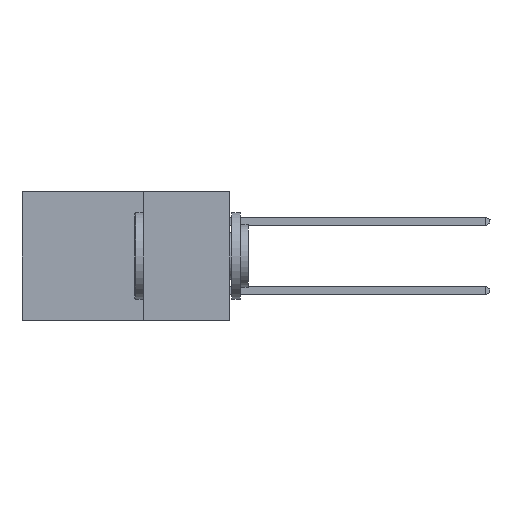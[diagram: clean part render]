
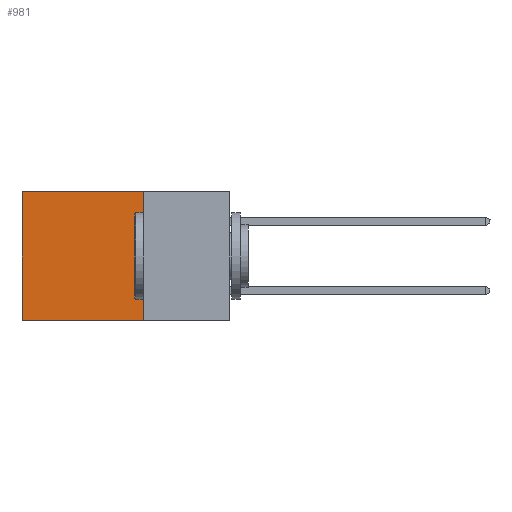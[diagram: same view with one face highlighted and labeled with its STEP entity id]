
A CAD part, left-side view. The second image highlights one B-rep face of the part: STEP entity #981.
In plain terms, the highlighted planar face has unit normal (-1, 0, 0).
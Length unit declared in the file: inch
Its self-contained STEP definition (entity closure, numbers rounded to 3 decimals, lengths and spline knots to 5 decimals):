
#30 = VERTEX_POINT ( 'NONE', #6367 ) ;
#65 = ORIENTED_EDGE ( 'NONE', *, *, #372, .T. ) ;
#151 = EDGE_CURVE ( 'NONE', #30, #8130, #11685, .T. ) ;
#372 = EDGE_CURVE ( 'NONE', #10210, #1152, #1036, .T. ) ;
#981 = ADVANCED_FACE ( 'NONE', ( #9003 ), #9372, .F. ) ;
#1036 = LINE ( 'NONE', #8754, #11535 ) ;
#1152 = VERTEX_POINT ( 'NONE', #12771 ) ;
#1383 = DIRECTION ( 'NONE',  ( 1., 0., 0. ) ) ;
#2819 = ORIENTED_EDGE ( 'NONE', *, *, #151, .F. ) ;
#3167 = ORIENTED_EDGE ( 'NONE', *, *, #12332, .F. ) ;
#3354 = DIRECTION ( 'NONE',  ( 0., 1., 0. ) ) ;
#3835 = CARTESIAN_POINT ( 'NONE',  ( 0.2615, 0.6, 0. ) ) ;
#4672 = CARTESIAN_POINT ( 'NONE',  ( 0.2615, 0.25, -0.37 ) ) ;
#4907 = VECTOR ( 'NONE', #12659, 39.37008 ) ;
#4984 = DIRECTION ( 'NONE',  ( 0., 0., -1. ) ) ;
#6367 = CARTESIAN_POINT ( 'NONE',  ( 0.2615, 0.25, 0. ) ) ;
#6370 = DIRECTION ( 'NONE',  ( 0., 0., -1. ) ) ;
#7176 = EDGE_LOOP ( 'NONE', ( #65, #3167, #2819, #11914 ) ) ;
#8130 = VERTEX_POINT ( 'NONE', #11707 ) ;
#8233 = CARTESIAN_POINT ( 'NONE',  ( 0.2615, 0.25, -0.37 ) ) ;
#8336 = LINE ( 'NONE', #10270, #12030 ) ;
#8754 = CARTESIAN_POINT ( 'NONE',  ( 0.2615, 0.6, -0.37 ) ) ;
#8954 = VECTOR ( 'NONE', #3354, 39.37008 ) ;
#9003 = FACE_OUTER_BOUND ( 'NONE', #7176, .T. ) ;
#9332 = LINE ( 'NONE', #8233, #8954 ) ;
#9372 = PLANE ( 'NONE',  #11803 ) ;
#9629 = CARTESIAN_POINT ( 'NONE',  ( 0.2615, 0.25, -0.37 ) ) ;
#10210 = VERTEX_POINT ( 'NONE', #3835 ) ;
#10270 = CARTESIAN_POINT ( 'NONE',  ( 0.2615, 0.25, 0. ) ) ;
#10524 = DIRECTION ( 'NONE',  ( 0., 1., 0. ) ) ;
#11451 = EDGE_CURVE ( 'NONE', #30, #10210, #8336, .T. ) ;
#11535 = VECTOR ( 'NONE', #4984, 39.37008 ) ;
#11685 = LINE ( 'NONE', #9629, #4907 ) ;
#11707 = CARTESIAN_POINT ( 'NONE',  ( 0.2615, 0.25, -0.37 ) ) ;
#11803 = AXIS2_PLACEMENT_3D ( 'NONE', #4672, #1383, #6370 ) ;
#11914 = ORIENTED_EDGE ( 'NONE', *, *, #11451, .T. ) ;
#12030 = VECTOR ( 'NONE', #10524, 39.37008 ) ;
#12332 = EDGE_CURVE ( 'NONE', #8130, #1152, #9332, .T. ) ;
#12659 = DIRECTION ( 'NONE',  ( 0., 0., -1. ) ) ;
#12771 = CARTESIAN_POINT ( 'NONE',  ( 0.2615, 0.6, -0.37 ) ) ;
